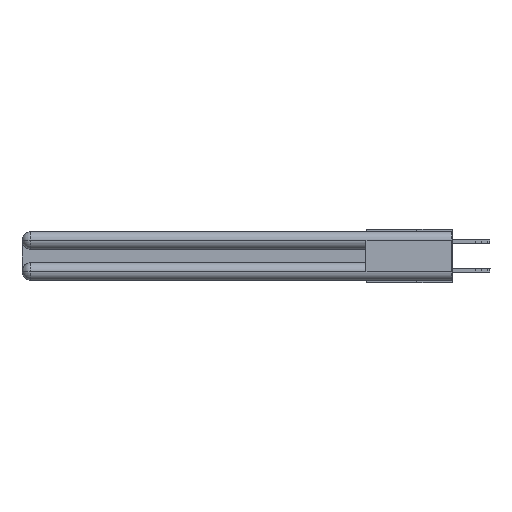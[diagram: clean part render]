
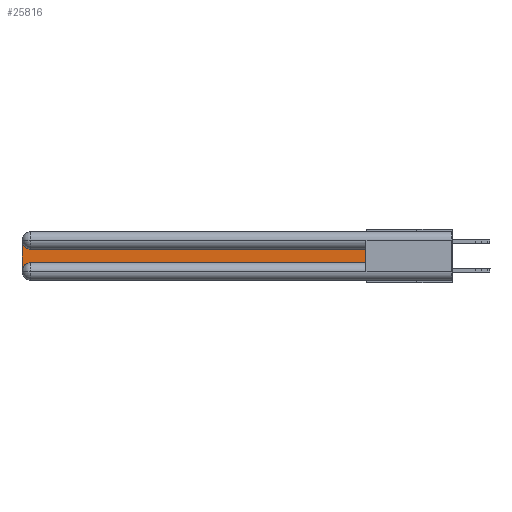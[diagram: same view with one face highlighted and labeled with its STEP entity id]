
A CAD part, left-side view. The second image highlights one B-rep face of the part: STEP entity #25816.
In plain terms, the highlighted planar face has unit normal (-1, 0, 0).
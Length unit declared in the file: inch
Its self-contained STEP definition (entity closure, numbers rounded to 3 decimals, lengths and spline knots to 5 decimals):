
#760 = VECTOR ( 'NONE', #9385, 39.37008 ) ;
#767 = CARTESIAN_POINT ( 'NONE',  ( 0.075, 3., -0.1225 ) ) ;
#855 = DIRECTION ( 'NONE',  ( 0., 1., 0. ) ) ;
#1744 = EDGE_CURVE ( 'NONE', #24453, #6609, #11382, .T. ) ;
#3226 = EDGE_CURVE ( 'NONE', #4101, #9885, #21323, .T. ) ;
#3413 = DIRECTION ( 'NONE',  ( 0., 0., -1. ) ) ;
#4016 = EDGE_LOOP ( 'NONE', ( #5788, #12091, #7833, #5545, #8270, #23419 ) ) ;
#4101 = VERTEX_POINT ( 'NONE', #19006 ) ;
#4228 = AXIS2_PLACEMENT_3D ( 'NONE', #9029, #23908, #9125 ) ;
#4721 = PLANE ( 'NONE',  #21343 ) ;
#5026 = FACE_OUTER_BOUND ( 'NONE', #4016, .T. ) ;
#5545 = ORIENTED_EDGE ( 'NONE', *, *, #3226, .T. ) ;
#5788 = ORIENTED_EDGE ( 'NONE', *, *, #1744, .T. ) ;
#5865 = CARTESIAN_POINT ( 'NONE',  ( 0.075, 0.6, -0.2175 ) ) ;
#6609 = VERTEX_POINT ( 'NONE', #27107 ) ;
#6874 = EDGE_CURVE ( 'NONE', #9885, #24145, #7319, .T. ) ;
#6914 = DIRECTION ( 'NONE',  ( 0., 0., -1. ) ) ;
#7186 = CARTESIAN_POINT ( 'NONE',  ( 0.075, 0.6, -0.1225 ) ) ;
#7319 = LINE ( 'NONE', #13201, #11990 ) ;
#7438 = CARTESIAN_POINT ( 'NONE',  ( 0.075, 0.6, -0.2175 ) ) ;
#7833 = ORIENTED_EDGE ( 'NONE', *, *, #19022, .T. ) ;
#7992 = CARTESIAN_POINT ( 'NONE',  ( 0.075, 2.94, -0.0625 ) ) ;
#8270 = ORIENTED_EDGE ( 'NONE', *, *, #6874, .T. ) ;
#9029 = CARTESIAN_POINT ( 'NONE',  ( 0.075, 2.94, -0.2775 ) ) ;
#9125 = DIRECTION ( 'NONE',  ( 0., 0., -1. ) ) ;
#9385 = DIRECTION ( 'NONE',  ( 0., 0., 1. ) ) ;
#9885 = VERTEX_POINT ( 'NONE', #21982 ) ;
#9943 = CARTESIAN_POINT ( 'NONE',  ( 0.075, 0.6, -0.1225 ) ) ;
#11382 = LINE ( 'NONE', #7186, #22393 ) ;
#11990 = VECTOR ( 'NONE', #15333, 39.37008 ) ;
#12091 = ORIENTED_EDGE ( 'NONE', *, *, #26071, .T. ) ;
#12535 = LINE ( 'NONE', #20979, #15188 ) ;
#13201 = CARTESIAN_POINT ( 'NONE',  ( 0.075, 0.6, -0.2175 ) ) ;
#14121 = DIRECTION ( 'NONE',  ( 1., 0., 0. ) ) ;
#15188 = VECTOR ( 'NONE', #17155, 39.37008 ) ;
#15333 = DIRECTION ( 'NONE',  ( 0., -1., 0. ) ) ;
#17155 = DIRECTION ( 'NONE',  ( 0., 0., -1. ) ) ;
#18668 = LINE ( 'NONE', #7438, #760 ) ;
#19006 = CARTESIAN_POINT ( 'NONE',  ( 0.075, 3., -0.2775 ) ) ;
#19022 = EDGE_CURVE ( 'NONE', #20539, #4101, #12535, .T. ) ;
#19936 = AXIS2_PLACEMENT_3D ( 'NONE', #7992, #14121, #3413 ) ;
#20539 = VERTEX_POINT ( 'NONE', #24664 ) ;
#20979 = CARTESIAN_POINT ( 'NONE',  ( 0.075, 3., -0.2175 ) ) ;
#21323 = CIRCLE ( 'NONE', #4228, 0.06 ) ;
#21343 = AXIS2_PLACEMENT_3D ( 'NONE', #767, #23720, #6914 ) ;
#21982 = CARTESIAN_POINT ( 'NONE',  ( 0.075, 2.94, -0.2175 ) ) ;
#22393 = VECTOR ( 'NONE', #855, 39.37008 ) ;
#23419 = ORIENTED_EDGE ( 'NONE', *, *, #25965, .T. ) ;
#23720 = DIRECTION ( 'NONE',  ( 1., 0., 0. ) ) ;
#23908 = DIRECTION ( 'NONE',  ( 1., 0., 0. ) ) ;
#24145 = VERTEX_POINT ( 'NONE', #5865 ) ;
#24453 = VERTEX_POINT ( 'NONE', #9943 ) ;
#24583 = CIRCLE ( 'NONE', #19936, 0.06 ) ;
#24664 = CARTESIAN_POINT ( 'NONE',  ( 0.075, 3., -0.0625 ) ) ;
#25816 = ADVANCED_FACE ( 'NONE', ( #5026 ), #4721, .F. ) ;
#25965 = EDGE_CURVE ( 'NONE', #24145, #24453, #18668, .T. ) ;
#26071 = EDGE_CURVE ( 'NONE', #6609, #20539, #24583, .T. ) ;
#27107 = CARTESIAN_POINT ( 'NONE',  ( 0.075, 2.94, -0.1225 ) ) ;
